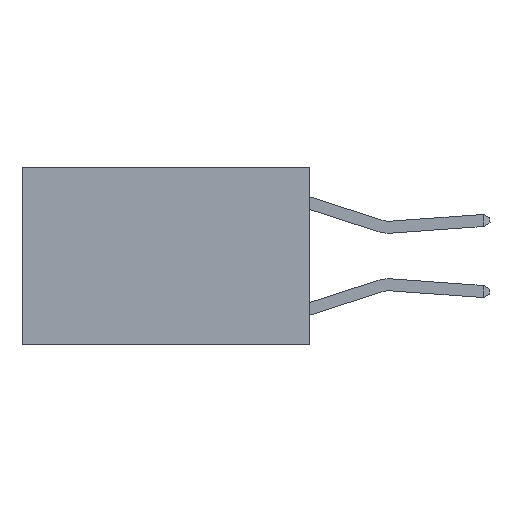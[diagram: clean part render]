
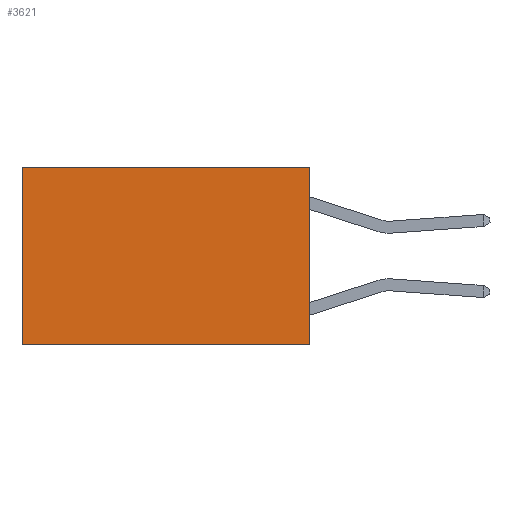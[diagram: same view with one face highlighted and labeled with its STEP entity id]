
A CAD part, left-side view. The second image highlights one B-rep face of the part: STEP entity #3621.
In plain terms, the highlighted planar face has unit normal (-1, 0, 0).
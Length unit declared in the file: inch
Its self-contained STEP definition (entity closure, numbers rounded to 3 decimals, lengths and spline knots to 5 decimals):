
#32 = LINE ( 'NONE', #370, #427 ) ;
#152 = VERTEX_POINT ( 'NONE', #1076 ) ;
#370 = CARTESIAN_POINT ( 'NONE',  ( 0.2625, 0.6, 0. ) ) ;
#404 = ORIENTED_EDGE ( 'NONE', *, *, #6438, .T. ) ;
#427 = VECTOR ( 'NONE', #483, 39.37008 ) ;
#448 = ORIENTED_EDGE ( 'NONE', *, *, #6520, .F. ) ;
#483 = DIRECTION ( 'NONE',  ( 0., 0., -1. ) ) ;
#995 = VECTOR ( 'NONE', #7085, 39.37008 ) ;
#1076 = CARTESIAN_POINT ( 'NONE',  ( 0.2625, 0.6, 0. ) ) ;
#1241 = ORIENTED_EDGE ( 'NONE', *, *, #5335, .F. ) ;
#1247 = AXIS2_PLACEMENT_3D ( 'NONE', #6316, #6247, #6129 ) ;
#1290 = LINE ( 'NONE', #5217, #995 ) ;
#2171 = CARTESIAN_POINT ( 'NONE',  ( 0.2625, 0., 0. ) ) ;
#2251 = VERTEX_POINT ( 'NONE', #4561 ) ;
#2961 = VERTEX_POINT ( 'NONE', #5836 ) ;
#3331 = FACE_OUTER_BOUND ( 'NONE', #5546, .T. ) ;
#3557 = ORIENTED_EDGE ( 'NONE', *, *, #6341, .T. ) ;
#3621 = ADVANCED_FACE ( 'NONE', ( #3331 ), #6515, .F. ) ;
#3694 = DIRECTION ( 'NONE',  ( 0., 0., -1. ) ) ;
#4095 = LINE ( 'NONE', #6396, #5040 ) ;
#4561 = CARTESIAN_POINT ( 'NONE',  ( 0.2625, 0., 0. ) ) ;
#5040 = VECTOR ( 'NONE', #6373, 39.37008 ) ;
#5177 = VERTEX_POINT ( 'NONE', #6833 ) ;
#5217 = CARTESIAN_POINT ( 'NONE',  ( 0.2625, 0., 0. ) ) ;
#5335 = EDGE_CURVE ( 'NONE', #5177, #2961, #4095, .T. ) ;
#5546 = EDGE_LOOP ( 'NONE', ( #3557, #1241, #448, #404 ) ) ;
#5836 = CARTESIAN_POINT ( 'NONE',  ( 0.2625, 0.6, -0.37 ) ) ;
#6129 = DIRECTION ( 'NONE',  ( 0., 0., -1. ) ) ;
#6247 = DIRECTION ( 'NONE',  ( 1., 0., 0. ) ) ;
#6316 = CARTESIAN_POINT ( 'NONE',  ( 0.2625, 0., 0. ) ) ;
#6341 = EDGE_CURVE ( 'NONE', #152, #2961, #32, .T. ) ;
#6373 = DIRECTION ( 'NONE',  ( 0., 1., 0. ) ) ;
#6396 = CARTESIAN_POINT ( 'NONE',  ( 0.2625, 0., -0.37 ) ) ;
#6438 = EDGE_CURVE ( 'NONE', #2251, #152, #1290, .T. ) ;
#6515 = PLANE ( 'NONE',  #1247 ) ;
#6520 = EDGE_CURVE ( 'NONE', #2251, #5177, #6890, .T. ) ;
#6588 = VECTOR ( 'NONE', #3694, 39.37008 ) ;
#6833 = CARTESIAN_POINT ( 'NONE',  ( 0.2625, 0., -0.37 ) ) ;
#6890 = LINE ( 'NONE', #2171, #6588 ) ;
#7085 = DIRECTION ( 'NONE',  ( 0., 1., 0. ) ) ;
